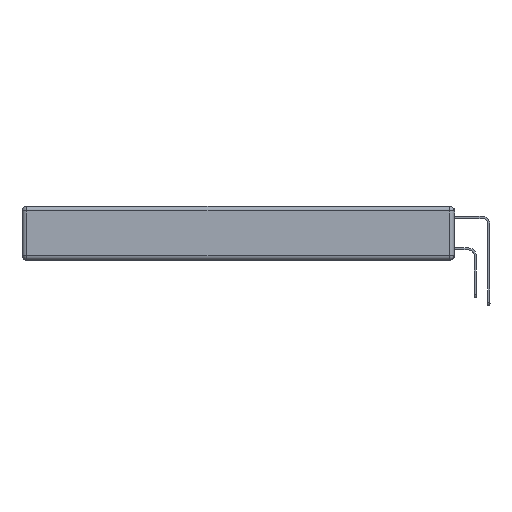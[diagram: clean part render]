
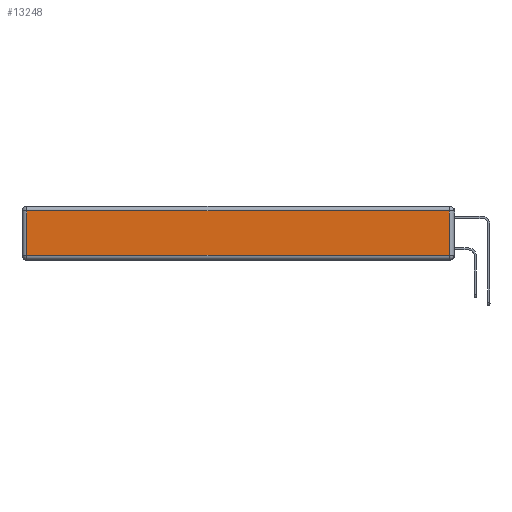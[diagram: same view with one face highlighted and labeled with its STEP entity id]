
A CAD part, left-side view. The second image highlights one B-rep face of the part: STEP entity #13248.
In plain terms, the highlighted planar face has unit normal (-1, 0, 0).
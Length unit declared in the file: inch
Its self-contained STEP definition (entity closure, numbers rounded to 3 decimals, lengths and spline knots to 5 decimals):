
#529 = VECTOR ( 'NONE', #9082, 39.37008 ) ;
#656 = VECTOR ( 'NONE', #17353, 39.37008 ) ;
#954 = LINE ( 'NONE', #2444, #14447 ) ;
#2426 = LINE ( 'NONE', #7906, #17011 ) ;
#2444 = CARTESIAN_POINT ( 'NONE',  ( 0., 0., -0.313 ) ) ;
#2541 = LINE ( 'NONE', #9955, #656 ) ;
#2566 = AXIS2_PLACEMENT_3D ( 'NONE', #19100, #19453, #21029 ) ;
#3044 = EDGE_CURVE ( 'NONE', #20175, #10100, #2541, .T. ) ;
#7906 = CARTESIAN_POINT ( 'NONE',  ( 0., 0.03, -0.343 ) ) ;
#8504 = DIRECTION ( 'NONE',  ( 0., -1., 0. ) ) ;
#9082 = DIRECTION ( 'NONE',  ( 0., 0., -1. ) ) ;
#9335 = LINE ( 'NONE', #23861, #529 ) ;
#9422 = CARTESIAN_POINT ( 'NONE',  ( 0., 0.03, -0.313 ) ) ;
#9955 = CARTESIAN_POINT ( 'NONE',  ( 0., 2.75, -0.03 ) ) ;
#10020 = PLANE ( 'NONE',  #2566 ) ;
#10100 = VERTEX_POINT ( 'NONE', #18402 ) ;
#10788 = ORIENTED_EDGE ( 'NONE', *, *, #15409, .T. ) ;
#11162 = EDGE_LOOP ( 'NONE', ( #20256, #10788, #15928, #22225 ) ) ;
#11790 = VERTEX_POINT ( 'NONE', #9422 ) ;
#11828 = FACE_OUTER_BOUND ( 'NONE', #11162, .T. ) ;
#13248 = ADVANCED_FACE ( 'NONE', ( #11828 ), #10020, .T. ) ;
#13654 = CARTESIAN_POINT ( 'NONE',  ( 0., 2.72, -0.313 ) ) ;
#14447 = VECTOR ( 'NONE', #8504, 39.37008 ) ;
#15409 = EDGE_CURVE ( 'NONE', #11790, #20175, #2426, .T. ) ;
#15928 = ORIENTED_EDGE ( 'NONE', *, *, #3044, .T. ) ;
#17011 = VECTOR ( 'NONE', #19173, 39.37008 ) ;
#17353 = DIRECTION ( 'NONE',  ( 0., 1., 0. ) ) ;
#18174 = VERTEX_POINT ( 'NONE', #13654 ) ;
#18402 = CARTESIAN_POINT ( 'NONE',  ( 0., 2.72, -0.03 ) ) ;
#19049 = EDGE_CURVE ( 'NONE', #18174, #11790, #954, .T. ) ;
#19100 = CARTESIAN_POINT ( 'NONE',  ( 0., 0., -0.343 ) ) ;
#19173 = DIRECTION ( 'NONE',  ( 0., 0., 1. ) ) ;
#19453 = DIRECTION ( 'NONE',  ( -1., 0., 0. ) ) ;
#20175 = VERTEX_POINT ( 'NONE', #21769 ) ;
#20256 = ORIENTED_EDGE ( 'NONE', *, *, #19049, .T. ) ;
#21029 = DIRECTION ( 'NONE',  ( 0., 0., 1. ) ) ;
#21769 = CARTESIAN_POINT ( 'NONE',  ( 0., 0.03, -0.03 ) ) ;
#22225 = ORIENTED_EDGE ( 'NONE', *, *, #23794, .T. ) ;
#23794 = EDGE_CURVE ( 'NONE', #10100, #18174, #9335, .T. ) ;
#23861 = CARTESIAN_POINT ( 'NONE',  ( 0., 2.72, -0.343 ) ) ;
